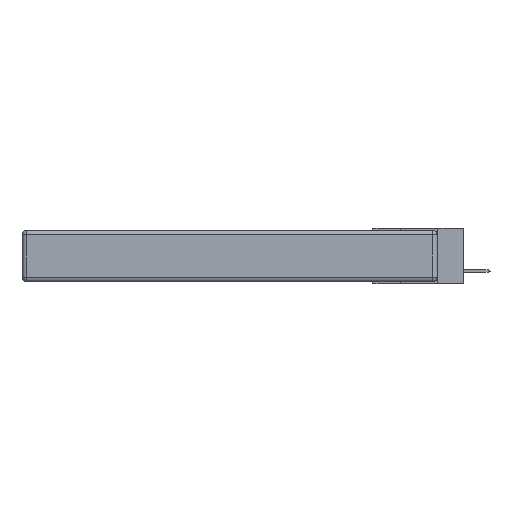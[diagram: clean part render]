
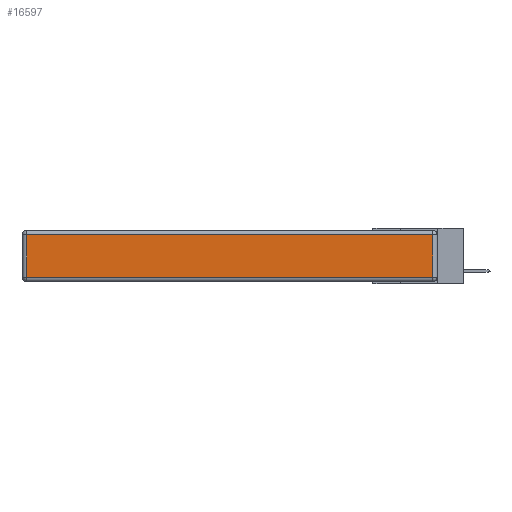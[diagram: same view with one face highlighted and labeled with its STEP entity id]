
A CAD part, left-side view. The second image highlights one B-rep face of the part: STEP entity #16597.
In plain terms, the highlighted planar face has unit normal (-1, 0, 0).
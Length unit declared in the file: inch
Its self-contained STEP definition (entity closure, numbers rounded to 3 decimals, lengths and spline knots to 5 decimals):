
#66 = EDGE_CURVE ( 'NONE', #9482, #16501, #5483, .T. ) ;
#843 = ORIENTED_EDGE ( 'NONE', *, *, #66, .T. ) ;
#1084 = EDGE_LOOP ( 'NONE', ( #4325, #9979, #843, #8482 ) ) ;
#1557 = FACE_OUTER_BOUND ( 'NONE', #1084, .T. ) ;
#2018 = LINE ( 'NONE', #11338, #7426 ) ;
#3279 = CARTESIAN_POINT ( 'NONE',  ( 0., 2.72, -0.313 ) ) ;
#4325 = ORIENTED_EDGE ( 'NONE', *, *, #9191, .T. ) ;
#4881 = AXIS2_PLACEMENT_3D ( 'NONE', #13748, #8174, #15467 ) ;
#5345 = DIRECTION ( 'NONE',  ( 0., 0., 1. ) ) ;
#5483 = LINE ( 'NONE', #23217, #13528 ) ;
#7426 = VECTOR ( 'NONE', #22371, 39.37008 ) ;
#8174 = DIRECTION ( 'NONE',  ( -1., 0., 0. ) ) ;
#8482 = ORIENTED_EDGE ( 'NONE', *, *, #9474, .T. ) ;
#9191 = EDGE_CURVE ( 'NONE', #18481, #18991, #2018, .T. ) ;
#9474 = EDGE_CURVE ( 'NONE', #16501, #18481, #20370, .T. ) ;
#9482 = VERTEX_POINT ( 'NONE', #17534 ) ;
#9685 = VECTOR ( 'NONE', #17303, 39.37008 ) ;
#9979 = ORIENTED_EDGE ( 'NONE', *, *, #20873, .T. ) ;
#11338 = CARTESIAN_POINT ( 'NONE',  ( 0., 0., -0.313 ) ) ;
#11394 = CARTESIAN_POINT ( 'NONE',  ( 0., 2.72, -0.03 ) ) ;
#11710 = PLANE ( 'NONE',  #4881 ) ;
#11946 = VECTOR ( 'NONE', #5345, 39.37008 ) ;
#13528 = VECTOR ( 'NONE', #21558, 39.37008 ) ;
#13748 = CARTESIAN_POINT ( 'NONE',  ( 0., 0., -0.343 ) ) ;
#14002 = CARTESIAN_POINT ( 'NONE',  ( 0., 0.03, -0.313 ) ) ;
#15467 = DIRECTION ( 'NONE',  ( 0., 0., 1. ) ) ;
#16501 = VERTEX_POINT ( 'NONE', #11394 ) ;
#16597 = ADVANCED_FACE ( 'NONE', ( #1557 ), #11710, .T. ) ;
#16898 = LINE ( 'NONE', #18204, #11946 ) ;
#17303 = DIRECTION ( 'NONE',  ( 0., 0., -1. ) ) ;
#17534 = CARTESIAN_POINT ( 'NONE',  ( 0., 0.03, -0.03 ) ) ;
#18204 = CARTESIAN_POINT ( 'NONE',  ( 0., 0.03, -0.343 ) ) ;
#18481 = VERTEX_POINT ( 'NONE', #3279 ) ;
#18964 = CARTESIAN_POINT ( 'NONE',  ( 0., 2.72, -0.343 ) ) ;
#18991 = VERTEX_POINT ( 'NONE', #14002 ) ;
#20370 = LINE ( 'NONE', #18964, #9685 ) ;
#20873 = EDGE_CURVE ( 'NONE', #18991, #9482, #16898, .T. ) ;
#21558 = DIRECTION ( 'NONE',  ( 0., 1., 0. ) ) ;
#22371 = DIRECTION ( 'NONE',  ( 0., -1., 0. ) ) ;
#23217 = CARTESIAN_POINT ( 'NONE',  ( 0., 2.75, -0.03 ) ) ;
